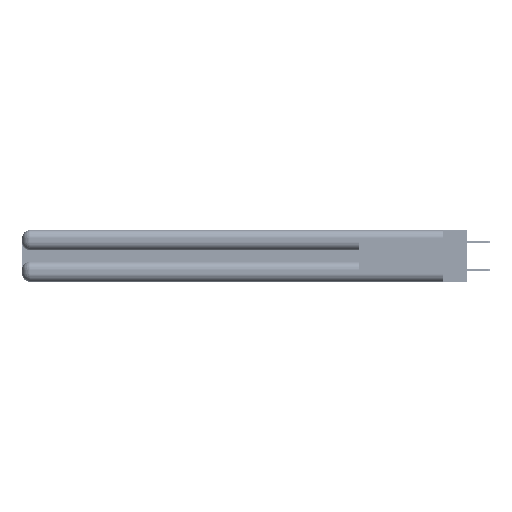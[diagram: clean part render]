
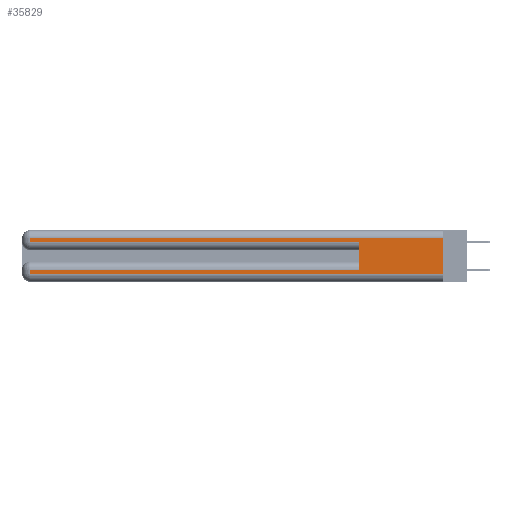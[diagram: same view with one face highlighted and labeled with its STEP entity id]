
A CAD part, left-side view. The second image highlights one B-rep face of the part: STEP entity #35829.
In plain terms, the highlighted planar face has unit normal (-1, 0, 0).
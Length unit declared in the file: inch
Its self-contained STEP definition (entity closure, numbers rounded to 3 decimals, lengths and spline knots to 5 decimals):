
#150 = VERTEX_POINT ( 'NONE', #46905 ) ;
#1005 = DIRECTION ( 'NONE',  ( 0., 0., -1. ) ) ;
#3836 = CARTESIAN_POINT ( 'NONE',  ( 0., 0., 0.06 ) ) ;
#4040 = LINE ( 'NONE', #47568, #38640 ) ;
#5473 = EDGE_CURVE ( 'NONE', #46836, #150, #26929, .T. ) ;
#6898 = CARTESIAN_POINT ( 'NONE',  ( 0., 0.6, 0.085 ) ) ;
#7910 = ORIENTED_EDGE ( 'NONE', *, *, #41436, .T. ) ;
#8060 = DIRECTION ( 'NONE',  ( 0., -1., 0. ) ) ;
#10293 = CARTESIAN_POINT ( 'NONE',  ( 0., 2.94, 0.37 ) ) ;
#11220 = AXIS2_PLACEMENT_3D ( 'NONE', #36298, #45380, #45755 ) ;
#14229 = EDGE_CURVE ( 'NONE', #40738, #34923, #22705, .T. ) ;
#14463 = CARTESIAN_POINT ( 'NONE',  ( 0., 2.94, 0.085 ) ) ;
#15827 = EDGE_LOOP ( 'NONE', ( #55754, #37521, #50644, #35442, #29972, #7910, #56053, #38230 ) ) ;
#16750 = EDGE_CURVE ( 'NONE', #32112, #25206, #19662, .T. ) ;
#18593 = DIRECTION ( 'NONE',  ( 0., 0., -1. ) ) ;
#19662 = LINE ( 'NONE', #36166, #46627 ) ;
#19912 = VECTOR ( 'NONE', #18593, 39.37008 ) ;
#22705 = LINE ( 'NONE', #10293, #19912 ) ;
#23307 = DIRECTION ( 'NONE',  ( 0., 0., 1. ) ) ;
#23624 = VERTEX_POINT ( 'NONE', #31208 ) ;
#24503 = VECTOR ( 'NONE', #43749, 39.37008 ) ;
#25206 = VERTEX_POINT ( 'NONE', #50912 ) ;
#25540 = VECTOR ( 'NONE', #23307, 39.37008 ) ;
#25886 = DIRECTION ( 'NONE',  ( 0., -1., 0. ) ) ;
#26638 = LINE ( 'NONE', #46489, #24503 ) ;
#26762 = FACE_OUTER_BOUND ( 'NONE', #15827, .T. ) ;
#26929 = LINE ( 'NONE', #54251, #25540 ) ;
#27461 = EDGE_CURVE ( 'NONE', #52330, #23624, #49099, .T. ) ;
#27468 = DIRECTION ( 'NONE',  ( 0., 1., 0. ) ) ;
#27979 = PLANE ( 'NONE',  #11220 ) ;
#29933 = CARTESIAN_POINT ( 'NONE',  ( 0., 2.94, 0.37 ) ) ;
#29972 = ORIENTED_EDGE ( 'NONE', *, *, #5473, .F. ) ;
#31208 = CARTESIAN_POINT ( 'NONE',  ( 0., 2.94, 0.285 ) ) ;
#32112 = VERTEX_POINT ( 'NONE', #46041 ) ;
#32605 = VECTOR ( 'NONE', #8060, 39.37008 ) ;
#34575 = DIRECTION ( 'NONE',  ( 0., 0., -1. ) ) ;
#34923 = VERTEX_POINT ( 'NONE', #56367 ) ;
#35442 = ORIENTED_EDGE ( 'NONE', *, *, #36807, .T. ) ;
#35829 = ADVANCED_FACE ( 'NONE', ( #26762 ), #27979, .F. ) ;
#36166 = CARTESIAN_POINT ( 'NONE',  ( 0., 0., 0.37 ) ) ;
#36298 = CARTESIAN_POINT ( 'NONE',  ( 0., 0., 0.37 ) ) ;
#36807 = EDGE_CURVE ( 'NONE', #23624, #150, #4040, .T. ) ;
#37521 = ORIENTED_EDGE ( 'NONE', *, *, #54591, .T. ) ;
#38230 = ORIENTED_EDGE ( 'NONE', *, *, #50966, .T. ) ;
#38640 = VECTOR ( 'NONE', #25886, 39.37008 ) ;
#39407 = VECTOR ( 'NONE', #34575, 39.37008 ) ;
#40738 = VERTEX_POINT ( 'NONE', #14463 ) ;
#41436 = EDGE_CURVE ( 'NONE', #46836, #40738, #48526, .T. ) ;
#43749 = DIRECTION ( 'NONE',  ( 0., 1., 0. ) ) ;
#45380 = DIRECTION ( 'NONE',  ( 1., 0., 0. ) ) ;
#45755 = DIRECTION ( 'NONE',  ( 0., 0., -1. ) ) ;
#46041 = CARTESIAN_POINT ( 'NONE',  ( 0., 0., 0.31 ) ) ;
#46489 = CARTESIAN_POINT ( 'NONE',  ( 0., 0., 0.31 ) ) ;
#46627 = VECTOR ( 'NONE', #1005, 39.37008 ) ;
#46836 = VERTEX_POINT ( 'NONE', #6898 ) ;
#46905 = CARTESIAN_POINT ( 'NONE',  ( 0., 0.6, 0.285 ) ) ;
#47123 = VECTOR ( 'NONE', #27468, 39.37008 ) ;
#47568 = CARTESIAN_POINT ( 'NONE',  ( 0., 0., 0.285 ) ) ;
#48526 = LINE ( 'NONE', #53946, #47123 ) ;
#49099 = LINE ( 'NONE', #29933, #39407 ) ;
#50030 = CARTESIAN_POINT ( 'NONE',  ( 0., 2.94, 0.31 ) ) ;
#50644 = ORIENTED_EDGE ( 'NONE', *, *, #27461, .T. ) ;
#50912 = CARTESIAN_POINT ( 'NONE',  ( 0., 0., 0.06 ) ) ;
#50966 = EDGE_CURVE ( 'NONE', #34923, #25206, #52637, .T. ) ;
#52330 = VERTEX_POINT ( 'NONE', #50030 ) ;
#52637 = LINE ( 'NONE', #3836, #32605 ) ;
#53946 = CARTESIAN_POINT ( 'NONE',  ( 0., 0., 0.085 ) ) ;
#54251 = CARTESIAN_POINT ( 'NONE',  ( 0., 0.6, 0.145 ) ) ;
#54591 = EDGE_CURVE ( 'NONE', #32112, #52330, #26638, .T. ) ;
#55754 = ORIENTED_EDGE ( 'NONE', *, *, #16750, .F. ) ;
#56053 = ORIENTED_EDGE ( 'NONE', *, *, #14229, .T. ) ;
#56367 = CARTESIAN_POINT ( 'NONE',  ( 0., 2.94, 0.06 ) ) ;
